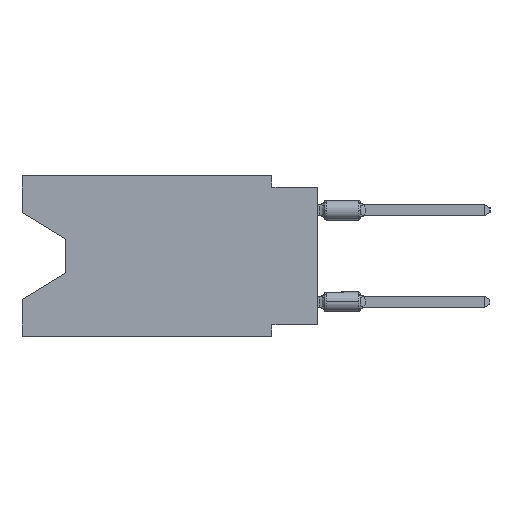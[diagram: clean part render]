
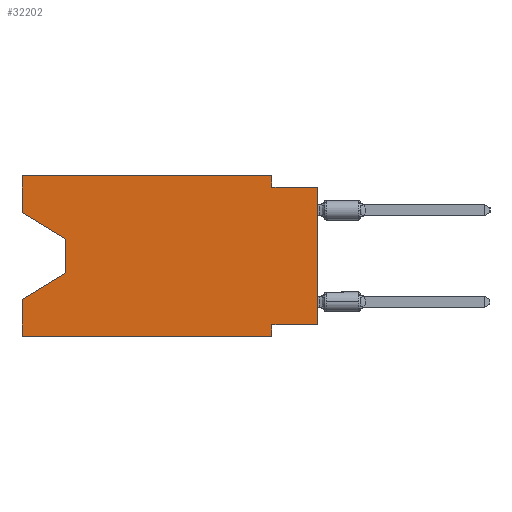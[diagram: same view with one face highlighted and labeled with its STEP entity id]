
A CAD part, left-side view. The second image highlights one B-rep face of the part: STEP entity #32202.
In plain terms, the highlighted planar face has unit normal (-1, 0, 0).
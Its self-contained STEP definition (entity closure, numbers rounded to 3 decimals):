
#84 = LINE ( 'NONE', #35323, #12313 ) ;
#1624 = VECTOR ( 'NONE', #65347, 1000. ) ;
#1845 = LINE ( 'NONE', #22819, #34184 ) ;
#1895 = VECTOR ( 'NONE', #15719, 1000. ) ;
#2717 = DIRECTION ( 'NONE',  ( 0., 0., -1. ) ) ;
#2786 = ORIENTED_EDGE ( 'NONE', *, *, #19834, .T. ) ;
#3546 = ORIENTED_EDGE ( 'NONE', *, *, #29878, .F. ) ;
#3808 = CARTESIAN_POINT ( 'NONE',  ( 0., 13.97, -5.385 ) ) ;
#4186 = ORIENTED_EDGE ( 'NONE', *, *, #18180, .T. ) ;
#4369 = DIRECTION ( 'NONE',  ( 0., -1., 0. ) ) ;
#4463 = EDGE_CURVE ( 'NONE', #22933, #56857, #64634, .T. ) ;
#4682 = EDGE_LOOP ( 'NONE', ( #2786, #21448, #59958, #10155, #4186, #40432, #59575, #37029, #36795, #3546, #14976, #60654 ) ) ;
#6348 = DIRECTION ( 'NONE',  ( 0., -1., 0. ) ) ;
#7708 = FACE_OUTER_BOUND ( 'NONE', #4682, .T. ) ;
#7830 = VECTOR ( 'NONE', #33085, 1000. ) ;
#8005 = EDGE_CURVE ( 'NONE', #17541, #21315, #32971, .T. ) ;
#8152 = LINE ( 'NONE', #28437, #7830 ) ;
#9795 = EDGE_CURVE ( 'NONE', #36907, #54113, #1845, .T. ) ;
#10155 = ORIENTED_EDGE ( 'NONE', *, *, #43642, .F. ) ;
#12287 = VERTEX_POINT ( 'NONE', #59948 ) ;
#12313 = VECTOR ( 'NONE', #60956, 1000. ) ;
#13781 = VECTOR ( 'NONE', #63210, 1000. ) ;
#14465 = CARTESIAN_POINT ( 'NONE',  ( 0., 2.54, -8.89 ) ) ;
#14976 = ORIENTED_EDGE ( 'NONE', *, *, #37501, .F. ) ;
#15719 = DIRECTION ( 'NONE',  ( 0., 0., 1. ) ) ;
#17466 = EDGE_CURVE ( 'NONE', #12287, #44270, #35370, .T. ) ;
#17541 = VERTEX_POINT ( 'NONE', #44369 ) ;
#18180 = EDGE_CURVE ( 'NONE', #47876, #43748, #40627, .T. ) ;
#19084 = CARTESIAN_POINT ( 'NONE',  ( 0., 16.383, 0. ) ) ;
#19834 = EDGE_CURVE ( 'NONE', #22933, #37854, #84, .T. ) ;
#20206 = CARTESIAN_POINT ( 'NONE',  ( 0., 16.383, 0. ) ) ;
#21315 = VERTEX_POINT ( 'NONE', #51176 ) ;
#21448 = ORIENTED_EDGE ( 'NONE', *, *, #57523, .T. ) ;
#21646 = CARTESIAN_POINT ( 'NONE',  ( 0., 2.54, -8.89 ) ) ;
#22819 = CARTESIAN_POINT ( 'NONE',  ( 0., 0., -0.635 ) ) ;
#22933 = VERTEX_POINT ( 'NONE', #28615 ) ;
#24892 = VERTEX_POINT ( 'NONE', #28870 ) ;
#25000 = CARTESIAN_POINT ( 'NONE',  ( 0., 16.383, 0. ) ) ;
#26475 = VECTOR ( 'NONE', #27984, 1000. ) ;
#27984 = DIRECTION ( 'NONE',  ( 0., 0., 1. ) ) ;
#27987 = CARTESIAN_POINT ( 'NONE',  ( 0., 0., -8.255 ) ) ;
#28437 = CARTESIAN_POINT ( 'NONE',  ( 0., 16.383, 0. ) ) ;
#28615 = CARTESIAN_POINT ( 'NONE',  ( 0., 16.383, -2.038 ) ) ;
#28870 = CARTESIAN_POINT ( 'NONE',  ( 0., 2.54, 0. ) ) ;
#29878 = EDGE_CURVE ( 'NONE', #24892, #36907, #63541, .T. ) ;
#32202 = ADVANCED_FACE ( 'NONE', ( #7708 ), #62622, .F. ) ;
#32321 = DIRECTION ( 'NONE',  ( 1., 0., 0. ) ) ;
#32971 = LINE ( 'NONE', #27987, #43528 ) ;
#33085 = DIRECTION ( 'NONE',  ( 0., 0., 1. ) ) ;
#33290 = DIRECTION ( 'NONE',  ( 0., 1., 0. ) ) ;
#34184 = VECTOR ( 'NONE', #42408, 1000. ) ;
#35323 = CARTESIAN_POINT ( 'NONE',  ( 0., 16.383, -2.038 ) ) ;
#35370 = LINE ( 'NONE', #3808, #1624 ) ;
#35865 = CARTESIAN_POINT ( 'NONE',  ( 0., 13.97, -3.505 ) ) ;
#36694 = VECTOR ( 'NONE', #6348, 1000. ) ;
#36795 = ORIENTED_EDGE ( 'NONE', *, *, #9795, .F. ) ;
#36907 = VERTEX_POINT ( 'NONE', #52359 ) ;
#37029 = ORIENTED_EDGE ( 'NONE', *, *, #65315, .T. ) ;
#37247 = CARTESIAN_POINT ( 'NONE',  ( 0., 2.54, 0. ) ) ;
#37501 = EDGE_CURVE ( 'NONE', #56857, #24892, #39946, .T. ) ;
#37854 = VERTEX_POINT ( 'NONE', #48540 ) ;
#39629 = CARTESIAN_POINT ( 'NONE',  ( 0., 0., -0.635 ) ) ;
#39946 = LINE ( 'NONE', #25000, #47103 ) ;
#40314 = CARTESIAN_POINT ( 'NONE',  ( 0., 16.383, -6.852 ) ) ;
#40432 = ORIENTED_EDGE ( 'NONE', *, *, #60392, .F. ) ;
#40627 = LINE ( 'NONE', #51253, #36694 ) ;
#41497 = LINE ( 'NONE', #35865, #62364 ) ;
#42408 = DIRECTION ( 'NONE',  ( 0., -1., 0. ) ) ;
#42919 = VECTOR ( 'NONE', #43214, 1000. ) ;
#43214 = DIRECTION ( 'NONE',  ( 0., 0., -1. ) ) ;
#43528 = VECTOR ( 'NONE', #33290, 1000. ) ;
#43642 = EDGE_CURVE ( 'NONE', #47876, #44270, #8152, .T. ) ;
#43748 = VERTEX_POINT ( 'NONE', #14465 ) ;
#44270 = VERTEX_POINT ( 'NONE', #40314 ) ;
#44369 = CARTESIAN_POINT ( 'NONE',  ( 0., 0., -8.255 ) ) ;
#47103 = VECTOR ( 'NONE', #4369, 1000. ) ;
#47876 = VERTEX_POINT ( 'NONE', #52711 ) ;
#48279 = CARTESIAN_POINT ( 'NONE',  ( 0., 16.383, 0. ) ) ;
#48365 = AXIS2_PLACEMENT_3D ( 'NONE', #48279, #32321, #2717 ) ;
#48540 = CARTESIAN_POINT ( 'NONE',  ( 0., 13.97, -3.505 ) ) ;
#51176 = CARTESIAN_POINT ( 'NONE',  ( 0., 2.54, -8.255 ) ) ;
#51253 = CARTESIAN_POINT ( 'NONE',  ( 0., 16.383, -8.89 ) ) ;
#52359 = CARTESIAN_POINT ( 'NONE',  ( 0., 2.54, -0.635 ) ) ;
#52711 = CARTESIAN_POINT ( 'NONE',  ( 0., 16.383, -8.89 ) ) ;
#54113 = VERTEX_POINT ( 'NONE', #39629 ) ;
#56857 = VERTEX_POINT ( 'NONE', #20206 ) ;
#57122 = DIRECTION ( 'NONE',  ( 0., 0., -1. ) ) ;
#57523 = EDGE_CURVE ( 'NONE', #37854, #12287, #41497, .T. ) ;
#59575 = ORIENTED_EDGE ( 'NONE', *, *, #8005, .F. ) ;
#59948 = CARTESIAN_POINT ( 'NONE',  ( 0., 13.97, -5.385 ) ) ;
#59958 = ORIENTED_EDGE ( 'NONE', *, *, #17466, .T. ) ;
#60392 = EDGE_CURVE ( 'NONE', #21315, #43748, #63202, .T. ) ;
#60654 = ORIENTED_EDGE ( 'NONE', *, *, #4463, .F. ) ;
#60956 = DIRECTION ( 'NONE',  ( 0., -0.855, -0.519 ) ) ;
#62364 = VECTOR ( 'NONE', #57122, 1000. ) ;
#62622 = PLANE ( 'NONE',  #48365 ) ;
#62914 = CARTESIAN_POINT ( 'NONE',  ( 0., 0., 0. ) ) ;
#63202 = LINE ( 'NONE', #21646, #42919 ) ;
#63210 = DIRECTION ( 'NONE',  ( 0., 0., -1. ) ) ;
#63247 = LINE ( 'NONE', #62914, #26475 ) ;
#63541 = LINE ( 'NONE', #37247, #13781 ) ;
#64634 = LINE ( 'NONE', #19084, #1895 ) ;
#65315 = EDGE_CURVE ( 'NONE', #17541, #54113, #63247, .T. ) ;
#65347 = DIRECTION ( 'NONE',  ( 0., 0.855, -0.519 ) ) ;
